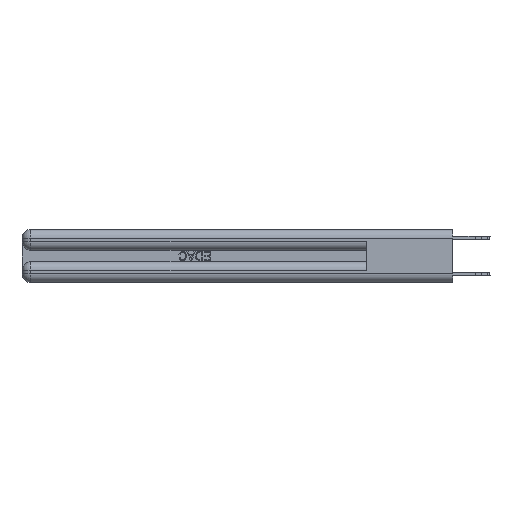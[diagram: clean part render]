
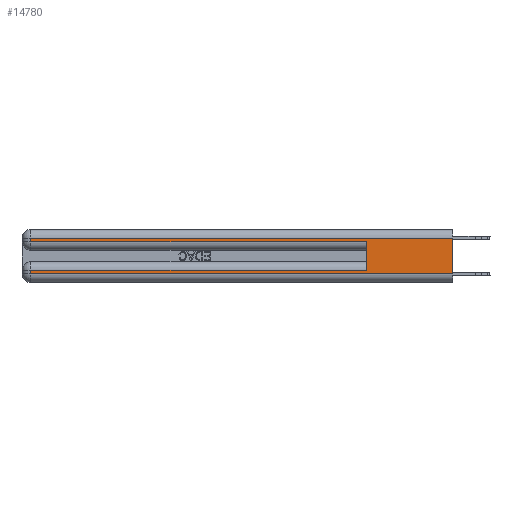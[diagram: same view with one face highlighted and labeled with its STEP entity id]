
A CAD part, left-side view. The second image highlights one B-rep face of the part: STEP entity #14780.
In plain terms, the highlighted planar face has unit normal (-1, 0, 0).
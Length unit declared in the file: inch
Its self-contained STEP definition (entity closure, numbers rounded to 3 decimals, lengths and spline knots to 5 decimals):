
#306 = CARTESIAN_POINT ( 'NONE',  ( 0., 0., 0.31 ) ) ;
#330 = VECTOR ( 'NONE', #17805, 39.37008 ) ;
#395 = VERTEX_POINT ( 'NONE', #1926 ) ;
#1607 = CARTESIAN_POINT ( 'NONE',  ( 0., 2.94, 0.37 ) ) ;
#1715 = CARTESIAN_POINT ( 'NONE',  ( 0., 0.6, 0.145 ) ) ;
#1888 = DIRECTION ( 'NONE',  ( 0., 0., -1. ) ) ;
#1926 = CARTESIAN_POINT ( 'NONE',  ( 0., 0.6, 0.085 ) ) ;
#2474 = PLANE ( 'NONE',  #29135 ) ;
#3317 = CARTESIAN_POINT ( 'NONE',  ( 0., 2.94, 0.285 ) ) ;
#3598 = CARTESIAN_POINT ( 'NONE',  ( 0., 0., 0.31 ) ) ;
#4536 = VECTOR ( 'NONE', #19628, 39.37008 ) ;
#5536 = VERTEX_POINT ( 'NONE', #5540 ) ;
#5540 = CARTESIAN_POINT ( 'NONE',  ( 0., 0.6, 0.285 ) ) ;
#5679 = EDGE_CURVE ( 'NONE', #19379, #17838, #8126, .T. ) ;
#6128 = ORIENTED_EDGE ( 'NONE', *, *, #23291, .T. ) ;
#6519 = VECTOR ( 'NONE', #10858, 39.37008 ) ;
#7258 = VERTEX_POINT ( 'NONE', #28191 ) ;
#7489 = CARTESIAN_POINT ( 'NONE',  ( 0., 0., 0.37 ) ) ;
#7690 = VERTEX_POINT ( 'NONE', #16851 ) ;
#7707 = ORIENTED_EDGE ( 'NONE', *, *, #22371, .T. ) ;
#8126 = LINE ( 'NONE', #22208, #4536 ) ;
#8337 = ORIENTED_EDGE ( 'NONE', *, *, #16455, .T. ) ;
#8440 = LINE ( 'NONE', #12827, #10962 ) ;
#8565 = LINE ( 'NONE', #1715, #330 ) ;
#8778 = VERTEX_POINT ( 'NONE', #25221 ) ;
#8793 = ORIENTED_EDGE ( 'NONE', *, *, #23838, .F. ) ;
#10616 = VECTOR ( 'NONE', #1888, 39.37008 ) ;
#10858 = DIRECTION ( 'NONE',  ( 0., 0., -1. ) ) ;
#10962 = VECTOR ( 'NONE', #22224, 39.37008 ) ;
#11650 = CARTESIAN_POINT ( 'NONE',  ( 0., 0., 0.06 ) ) ;
#12827 = CARTESIAN_POINT ( 'NONE',  ( 0., 0., 0.06 ) ) ;
#13253 = LINE ( 'NONE', #20692, #10616 ) ;
#14008 = VERTEX_POINT ( 'NONE', #3317 ) ;
#14780 = ADVANCED_FACE ( 'NONE', ( #18567 ), #2474, .F. ) ;
#15352 = VECTOR ( 'NONE', #15946, 39.37008 ) ;
#15946 = DIRECTION ( 'NONE',  ( 0., 1., 0. ) ) ;
#16149 = DIRECTION ( 'NONE',  ( 1., 0., 0. ) ) ;
#16350 = ORIENTED_EDGE ( 'NONE', *, *, #28975, .T. ) ;
#16455 = EDGE_CURVE ( 'NONE', #7258, #8778, #22823, .T. ) ;
#16548 = LINE ( 'NONE', #28167, #21569 ) ;
#16851 = CARTESIAN_POINT ( 'NONE',  ( 0., 2.94, 0.31 ) ) ;
#17272 = CARTESIAN_POINT ( 'NONE',  ( 0., 0., 0.285 ) ) ;
#17805 = DIRECTION ( 'NONE',  ( 0., 0., 1. ) ) ;
#17838 = VERTEX_POINT ( 'NONE', #11650 ) ;
#18567 = FACE_OUTER_BOUND ( 'NONE', #26489, .T. ) ;
#18644 = EDGE_CURVE ( 'NONE', #19379, #7690, #20638, .T. ) ;
#19379 = VERTEX_POINT ( 'NONE', #3598 ) ;
#19628 = DIRECTION ( 'NONE',  ( 0., 0., -1. ) ) ;
#19858 = DIRECTION ( 'NONE',  ( 0., -1., 0. ) ) ;
#20638 = LINE ( 'NONE', #306, #15352 ) ;
#20692 = CARTESIAN_POINT ( 'NONE',  ( 0., 2.94, 0.37 ) ) ;
#21569 = VECTOR ( 'NONE', #25781, 39.37008 ) ;
#22208 = CARTESIAN_POINT ( 'NONE',  ( 0., 0., 0.37 ) ) ;
#22224 = DIRECTION ( 'NONE',  ( 0., -1., 0. ) ) ;
#22371 = EDGE_CURVE ( 'NONE', #395, #7258, #16548, .T. ) ;
#22823 = LINE ( 'NONE', #1607, #6519 ) ;
#23211 = ORIENTED_EDGE ( 'NONE', *, *, #18644, .T. ) ;
#23291 = EDGE_CURVE ( 'NONE', #8778, #17838, #8440, .T. ) ;
#23838 = EDGE_CURVE ( 'NONE', #395, #5536, #8565, .T. ) ;
#24116 = VECTOR ( 'NONE', #19858, 39.37008 ) ;
#25221 = CARTESIAN_POINT ( 'NONE',  ( 0., 2.94, 0.06 ) ) ;
#25781 = DIRECTION ( 'NONE',  ( 0., 1., 0. ) ) ;
#25789 = ORIENTED_EDGE ( 'NONE', *, *, #27490, .T. ) ;
#26489 = EDGE_LOOP ( 'NONE', ( #27061, #23211, #16350, #25789, #8793, #7707, #8337, #6128 ) ) ;
#27061 = ORIENTED_EDGE ( 'NONE', *, *, #5679, .F. ) ;
#27490 = EDGE_CURVE ( 'NONE', #14008, #5536, #29166, .T. ) ;
#27778 = DIRECTION ( 'NONE',  ( 0., 0., -1. ) ) ;
#28167 = CARTESIAN_POINT ( 'NONE',  ( 0., 0., 0.085 ) ) ;
#28191 = CARTESIAN_POINT ( 'NONE',  ( 0., 2.94, 0.085 ) ) ;
#28975 = EDGE_CURVE ( 'NONE', #7690, #14008, #13253, .T. ) ;
#29135 = AXIS2_PLACEMENT_3D ( 'NONE', #7489, #16149, #27778 ) ;
#29166 = LINE ( 'NONE', #17272, #24116 ) ;
